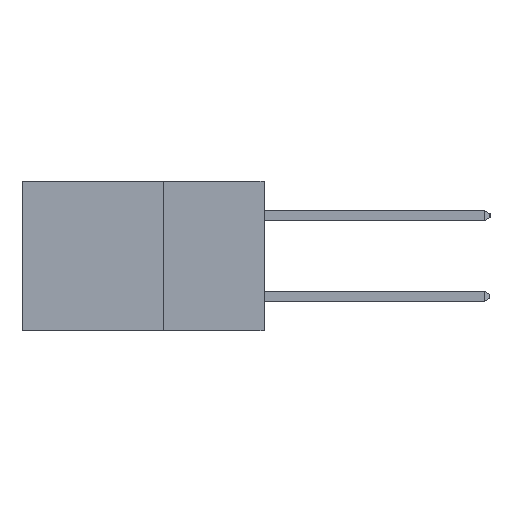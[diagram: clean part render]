
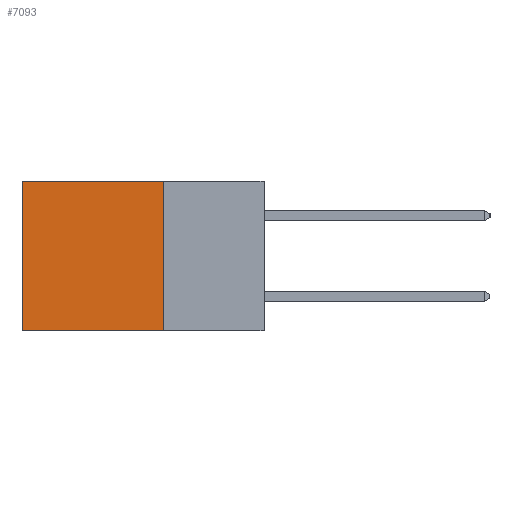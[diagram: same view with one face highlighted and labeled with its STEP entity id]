
A CAD part, left-side view. The second image highlights one B-rep face of the part: STEP entity #7093.
In plain terms, the highlighted planar face has unit normal (-1, 0, 0).
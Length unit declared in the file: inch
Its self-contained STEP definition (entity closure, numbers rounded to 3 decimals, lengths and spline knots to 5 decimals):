
#127 = VECTOR ( 'NONE', #2711, 39.37008 ) ;
#380 = EDGE_LOOP ( 'NONE', ( #10596, #8155, #3408, #6671 ) ) ;
#426 = CARTESIAN_POINT ( 'NONE',  ( 0.2615, 0.25, 0. ) ) ;
#484 = VERTEX_POINT ( 'NONE', #12735 ) ;
#841 = DIRECTION ( 'NONE',  ( 1., 0., 0. ) ) ;
#986 = FACE_OUTER_BOUND ( 'NONE', #380, .T. ) ;
#1109 = PLANE ( 'NONE',  #7386 ) ;
#1147 = VERTEX_POINT ( 'NONE', #12979 ) ;
#1488 = VERTEX_POINT ( 'NONE', #4770 ) ;
#2055 = CARTESIAN_POINT ( 'NONE',  ( 0.2615, 0.25, -0.37 ) ) ;
#2485 = EDGE_CURVE ( 'NONE', #1488, #1147, #3715, .T. ) ;
#2711 = DIRECTION ( 'NONE',  ( 0., 0., -1. ) ) ;
#3215 = EDGE_CURVE ( 'NONE', #484, #12968, #3419, .T. ) ;
#3265 = DIRECTION ( 'NONE',  ( 0., 1., 0. ) ) ;
#3408 = ORIENTED_EDGE ( 'NONE', *, *, #3215, .F. ) ;
#3419 = LINE ( 'NONE', #6634, #7146 ) ;
#3715 = LINE ( 'NONE', #11968, #127 ) ;
#4770 = CARTESIAN_POINT ( 'NONE',  ( 0.2615, 0.6, 0. ) ) ;
#4940 = DIRECTION ( 'NONE',  ( 0., 0., -1. ) ) ;
#5331 = LINE ( 'NONE', #12651, #6333 ) ;
#5900 = EDGE_CURVE ( 'NONE', #12968, #1147, #5331, .T. ) ;
#5994 = EDGE_CURVE ( 'NONE', #484, #1488, #8787, .T. ) ;
#6333 = VECTOR ( 'NONE', #3265, 39.37008 ) ;
#6634 = CARTESIAN_POINT ( 'NONE',  ( 0.2615, 0.25, -0.37 ) ) ;
#6671 = ORIENTED_EDGE ( 'NONE', *, *, #5994, .T. ) ;
#6998 = VECTOR ( 'NONE', #12853, 39.37008 ) ;
#7093 = ADVANCED_FACE ( 'NONE', ( #986 ), #1109, .F. ) ;
#7146 = VECTOR ( 'NONE', #12667, 39.37008 ) ;
#7386 = AXIS2_PLACEMENT_3D ( 'NONE', #2055, #841, #4940 ) ;
#8155 = ORIENTED_EDGE ( 'NONE', *, *, #5900, .F. ) ;
#8787 = LINE ( 'NONE', #426, #6998 ) ;
#10596 = ORIENTED_EDGE ( 'NONE', *, *, #2485, .T. ) ;
#11631 = CARTESIAN_POINT ( 'NONE',  ( 0.2615, 0.25, -0.37 ) ) ;
#11968 = CARTESIAN_POINT ( 'NONE',  ( 0.2615, 0.6, -0.37 ) ) ;
#12651 = CARTESIAN_POINT ( 'NONE',  ( 0.2615, 0.25, -0.37 ) ) ;
#12667 = DIRECTION ( 'NONE',  ( 0., 0., -1. ) ) ;
#12735 = CARTESIAN_POINT ( 'NONE',  ( 0.2615, 0.25, 0. ) ) ;
#12853 = DIRECTION ( 'NONE',  ( 0., 1., 0. ) ) ;
#12968 = VERTEX_POINT ( 'NONE', #11631 ) ;
#12979 = CARTESIAN_POINT ( 'NONE',  ( 0.2615, 0.6, -0.37 ) ) ;
